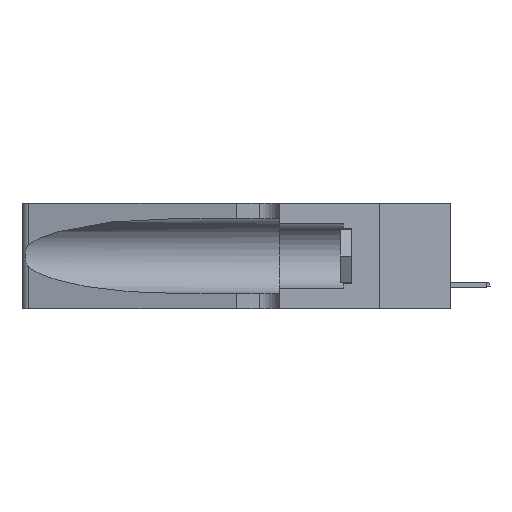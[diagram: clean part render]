
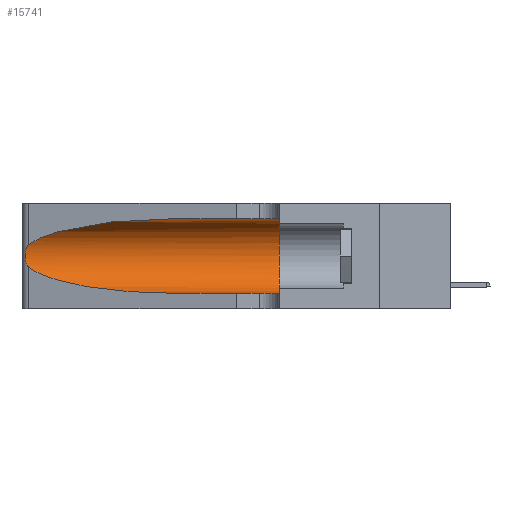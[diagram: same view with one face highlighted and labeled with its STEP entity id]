
A CAD part, left-side view. The second image highlights one B-rep face of the part: STEP entity #15741.
In plain terms, the highlighted cylindrical face has radius 3.308 mm (diameter 6.617 mm), a partial arc.
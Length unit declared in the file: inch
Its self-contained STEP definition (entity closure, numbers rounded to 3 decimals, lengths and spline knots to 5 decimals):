
#91 = CARTESIAN_POINT ( 'NONE',  ( 0.25856, 1.23593, 0.16098 ) ) ;
#823 = EDGE_CURVE ( 'NONE', #9768, #18796, #1128, .T. ) ;
#1128 =( BOUNDED_CURVE ( )  B_SPLINE_CURVE ( 3, ( #13065, #19869, #8360, #16939 ),
 .UNSPECIFIED., .F., .F. ) 
 B_SPLINE_CURVE_WITH_KNOTS ( ( 4, 4 ),
 ( 3.44316, 4.71239 ),
 .UNSPECIFIED. ) 
 CURVE ( )  GEOMETRIC_REPRESENTATION_ITEM ( )  RATIONAL_B_SPLINE_CURVE ( ( 1., 0.87, 0.87, 1. ) ) 
 REPRESENTATION_ITEM ( '' )  );
#1244 = EDGE_LOOP ( 'NONE', ( #2364, #15746, #10966, #22035, #13757, #13897 ) ) ;
#1531 = CARTESIAN_POINT ( 'NONE',  ( 0.26018, 1.23835, 0.19895 ) ) ;
#1958 = CARTESIAN_POINT ( 'NONE',  ( 0.26075, 1.23896, 0.178 ) ) ;
#2205 = CARTESIAN_POINT ( 'NONE',  ( 0.18966, 0.96281, 0.31525 ) ) ;
#2364 = ORIENTED_EDGE ( 'NONE', *, *, #18053, .T. ) ;
#2885 = AXIS2_PLACEMENT_3D ( 'NONE', #10045, #21757, #18423 ) ;
#3204 = CARTESIAN_POINT ( 'NONE',  ( 0.25487, 1.22718, 0.14631 ) ) ;
#3234 = CIRCLE ( 'NONE', #2885, 0.13025 ) ;
#3275 = VERTEX_POINT ( 'NONE', #12734 ) ;
#3324 = EDGE_CURVE ( 'NONE', #11649, #5261, #3234, .T. ) ;
#3354 = CYLINDRICAL_SURFACE ( 'NONE', #15306, 0.13025 ) ;
#3399 = CARTESIAN_POINT ( 'NONE',  ( 0.25639, 1.23186, 0.15144 ) ) ;
#3468 = CARTESIAN_POINT ( 'NONE',  ( 0.1305, 1.61858, 0.185 ) ) ;
#3620 = CARTESIAN_POINT ( 'NONE',  ( 0.26075, 1.23896, 0.19203 ) ) ;
#3936 = CARTESIAN_POINT ( 'NONE',  ( 0.1305, 1.61858, 0.05475 ) ) ;
#5045 = CARTESIAN_POINT ( 'NONE',  ( 0.1305, 0.72297, 0.31525 ) ) ;
#5108 = EDGE_CURVE ( 'NONE', #3275, #9768, #8953, .T. ) ;
#5210 = CARTESIAN_POINT ( 'NONE',  ( 0.25787, 1.23484, 0.2124 ) ) ;
#5261 = VERTEX_POINT ( 'NONE', #18337 ) ;
#5375 = DIRECTION ( 'NONE',  ( 0., -1., 0. ) ) ;
#5690 =( BOUNDED_CURVE ( )  B_SPLINE_CURVE ( 3, ( #17913, #2205, #14034, #9449 ),
 .UNSPECIFIED., .F., .T. ) 
 B_SPLINE_CURVE_WITH_KNOTS ( ( 4, 4 ),
 ( 1.5708, 2.84003 ),
 .UNSPECIFIED. ) 
 CURVE ( )  GEOMETRIC_REPRESENTATION_ITEM ( )  RATIONAL_B_SPLINE_CURVE ( ( 1., 0.87, 0.87, 1. ) ) 
 REPRESENTATION_ITEM ( '' )  );
#6992 = DIRECTION ( 'NONE',  ( 0., 0., -1. ) ) ;
#7156 = CARTESIAN_POINT ( 'NONE',  ( 0.26017, 1.23833, 0.17102 ) ) ;
#7359 = LINE ( 'NONE', #3936, #18844 ) ;
#8360 = CARTESIAN_POINT ( 'NONE',  ( 0.18966, 0.96281, 0.05475 ) ) ;
#8953 = B_SPLINE_CURVE_WITH_KNOTS ( 'NONE', 3,
 ( #16896, #19011, #18908, #5210, #17330, #1531, #3620, #1958, #7156, #91, #20688, #3399, #13767, #10339 ),
 .UNSPECIFIED., .F., .F.,
 ( 4, 2, 2, 2, 2, 2, 4 ),
 ( 0., 0.00027, 0.00053, 0.00107, 0.0016, 0.00187, 0.00214 ),
 .UNSPECIFIED. ) ;
#9247 = VECTOR ( 'NONE', #20140, 39.37008 ) ;
#9449 = CARTESIAN_POINT ( 'NONE',  ( 0.25487, 1.22718, 0.22369 ) ) ;
#9768 = VERTEX_POINT ( 'NONE', #3204 ) ;
#10045 = CARTESIAN_POINT ( 'NONE',  ( 0.1305, 0.35, 0.185 ) ) ;
#10339 = CARTESIAN_POINT ( 'NONE',  ( 0.25487, 1.22718, 0.14631 ) ) ;
#10966 = ORIENTED_EDGE ( 'NONE', *, *, #823, .T. ) ;
#11336 = CARTESIAN_POINT ( 'NONE',  ( 0.1305, 0.35, 0.31525 ) ) ;
#11649 = VERTEX_POINT ( 'NONE', #11336 ) ;
#12734 = CARTESIAN_POINT ( 'NONE',  ( 0.25487, 1.22718, 0.22369 ) ) ;
#13065 = CARTESIAN_POINT ( 'NONE',  ( 0.25487, 1.22718, 0.14631 ) ) ;
#13515 = FACE_OUTER_BOUND ( 'NONE', #1244, .T. ) ;
#13757 = ORIENTED_EDGE ( 'NONE', *, *, #3324, .F. ) ;
#13767 = CARTESIAN_POINT ( 'NONE',  ( 0.25555, 1.22993, 0.14849 ) ) ;
#13897 = ORIENTED_EDGE ( 'NONE', *, *, #15465, .F. ) ;
#14034 = CARTESIAN_POINT ( 'NONE',  ( 0.2373, 1.15595, 0.28018 ) ) ;
#15306 = AXIS2_PLACEMENT_3D ( 'NONE', #3468, #5375, #6992 ) ;
#15465 = EDGE_CURVE ( 'NONE', #20657, #11649, #18556, .T. ) ;
#15731 = DIRECTION ( 'NONE',  ( 0., -1., 0. ) ) ;
#15741 = ADVANCED_FACE ( 'NONE', ( #13515 ), #3354, .F. ) ;
#15746 = ORIENTED_EDGE ( 'NONE', *, *, #5108, .T. ) ;
#16896 = CARTESIAN_POINT ( 'NONE',  ( 0.25487, 1.22718, 0.22369 ) ) ;
#16939 = CARTESIAN_POINT ( 'NONE',  ( 0.1305, 0.72297, 0.05475 ) ) ;
#17330 = CARTESIAN_POINT ( 'NONE',  ( 0.25854, 1.2359, 0.20912 ) ) ;
#17777 = EDGE_CURVE ( 'NONE', #18796, #5261, #7359, .T. ) ;
#17913 = CARTESIAN_POINT ( 'NONE',  ( 0.1305, 0.72297, 0.31525 ) ) ;
#18053 = EDGE_CURVE ( 'NONE', #20657, #3275, #5690, .T. ) ;
#18337 = CARTESIAN_POINT ( 'NONE',  ( 0.1305, 0.35, 0.05475 ) ) ;
#18423 = DIRECTION ( 'NONE',  ( 0., 0., 1. ) ) ;
#18556 = LINE ( 'NONE', #21897, #9247 ) ;
#18796 = VERTEX_POINT ( 'NONE', #21163 ) ;
#18844 = VECTOR ( 'NONE', #15731, 39.37008 ) ;
#18908 = CARTESIAN_POINT ( 'NONE',  ( 0.25639, 1.23184, 0.21858 ) ) ;
#19011 = CARTESIAN_POINT ( 'NONE',  ( 0.25555, 1.22994, 0.2215 ) ) ;
#19869 = CARTESIAN_POINT ( 'NONE',  ( 0.2373, 1.15595, 0.08982 ) ) ;
#20140 = DIRECTION ( 'NONE',  ( 0., -1., 0. ) ) ;
#20657 = VERTEX_POINT ( 'NONE', #5045 ) ;
#20688 = CARTESIAN_POINT ( 'NONE',  ( 0.25789, 1.23486, 0.15765 ) ) ;
#21163 = CARTESIAN_POINT ( 'NONE',  ( 0.1305, 0.72297, 0.05475 ) ) ;
#21757 = DIRECTION ( 'NONE',  ( 0., 1., 0. ) ) ;
#21897 = CARTESIAN_POINT ( 'NONE',  ( 0.1305, 1.61858, 0.31525 ) ) ;
#22035 = ORIENTED_EDGE ( 'NONE', *, *, #17777, .T. ) ;
